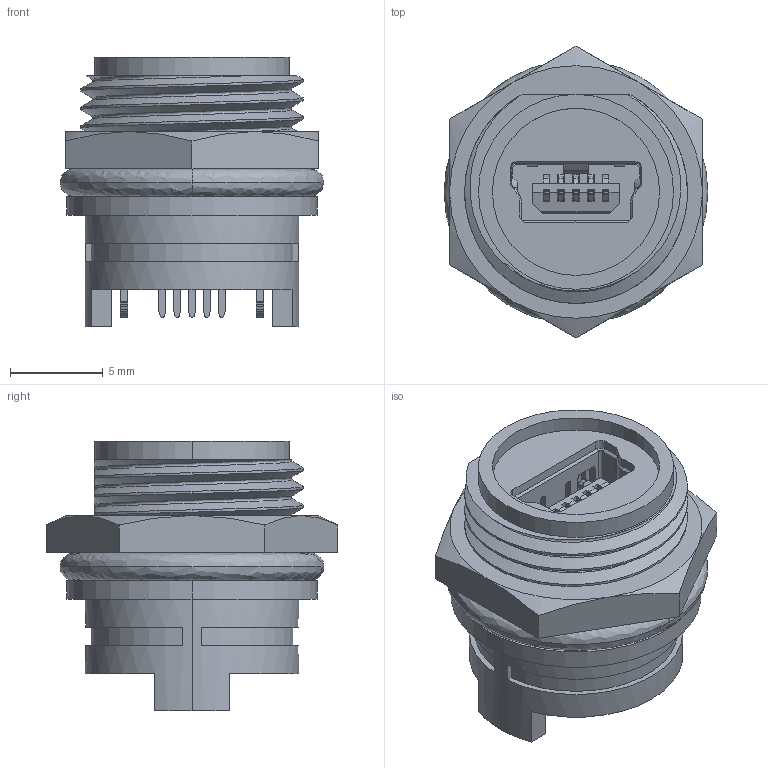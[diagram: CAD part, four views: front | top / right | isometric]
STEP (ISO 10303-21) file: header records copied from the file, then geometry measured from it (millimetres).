
FILE_DESCRIPTION (( 'STEP AP214' ), '1' );
FILE_NAME ('690-W05-660-044.STEP', '2021-04-12T21:05:16', ( '' ), ( '' ), 'SwSTEP 2.0', 'SolidWorks 2020', '' );
FILE_SCHEMA (( 'AUTOMOTIVE_DESIGN' ));
Length unit declared in the file: millimetre
Products named in the file (1): 690-W05-660-044
Bounding box: 14.2 x 15.7 x 14.5 mm (x, y, z)
Volume: 913.4 mm3; surface area: 2247.5 mm2
Topology: 1 solids, 2 shells, 885 faces, 2605 edges, 1701 vertices
Faces by surface type: plane 593, cylinder 235, bspline 43, cone 14
Entity records: 34776 total; most frequent: CARTESIAN_POINT 10146, ORIENTED_EDGE 5202, DIRECTION 4453, EDGE_CURVE 2601, VECTOR 1877, LINE 1877, VERTEX_POINT 1700, AXIS2_PLACEMENT_3D 1288
